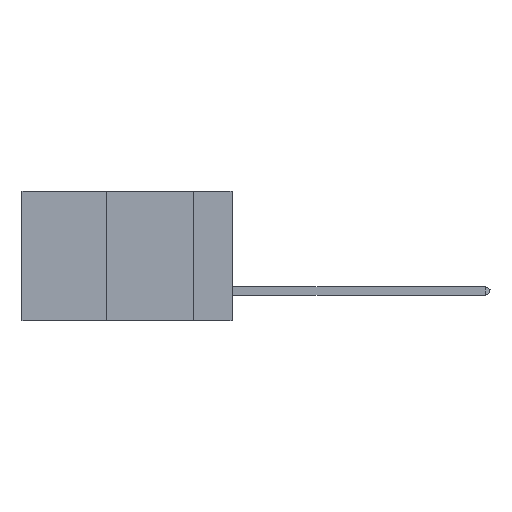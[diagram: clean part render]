
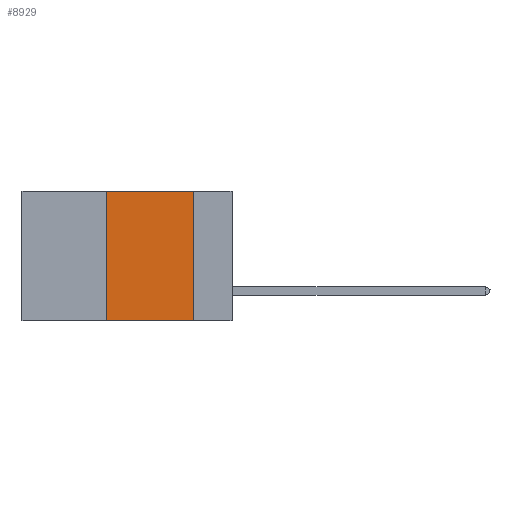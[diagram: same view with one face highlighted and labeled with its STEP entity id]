
A CAD part, left-side view. The second image highlights one B-rep face of the part: STEP entity #8929.
In plain terms, the highlighted planar face has unit normal (-1, 0, 0).
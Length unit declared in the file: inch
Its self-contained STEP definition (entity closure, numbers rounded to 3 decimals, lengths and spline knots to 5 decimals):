
#135 = CARTESIAN_POINT ( 'NONE',  ( 0., 0.36, 0. ) ) ;
#258 = DIRECTION ( 'NONE',  ( 0., 0., 1. ) ) ;
#318 = DIRECTION ( 'NONE',  ( 1., 0., 0. ) ) ;
#398 = VECTOR ( 'NONE', #1254, 39.37008 ) ;
#1254 = DIRECTION ( 'NONE',  ( 0., 0., -1. ) ) ;
#1463 = DIRECTION ( 'NONE',  ( 0., -1., 0. ) ) ;
#1629 = DIRECTION ( 'NONE',  ( 0., -1., 0. ) ) ;
#2200 = VECTOR ( 'NONE', #1629, 39.37008 ) ;
#2343 = ORIENTED_EDGE ( 'NONE', *, *, #4038, .F. ) ;
#2389 = VERTEX_POINT ( 'NONE', #10742 ) ;
#3340 = LINE ( 'NONE', #135, #8206 ) ;
#3611 = CARTESIAN_POINT ( 'NONE',  ( 0., 0.11, 0. ) ) ;
#3669 = VERTEX_POINT ( 'NONE', #8957 ) ;
#4038 = EDGE_CURVE ( 'NONE', #2389, #3669, #3340, .T. ) ;
#4509 = LINE ( 'NONE', #11048, #2200 ) ;
#4709 = AXIS2_PLACEMENT_3D ( 'NONE', #8963, #318, #8006 ) ;
#4723 = ORIENTED_EDGE ( 'NONE', *, *, #5851, .F. ) ;
#4861 = EDGE_LOOP ( 'NONE', ( #4723, #11963, #2343, #10831 ) ) ;
#5778 = EDGE_CURVE ( 'NONE', #3669, #8284, #5887, .T. ) ;
#5851 = EDGE_CURVE ( 'NONE', #8284, #12227, #9805, .T. ) ;
#5887 = LINE ( 'NONE', #7289, #8143 ) ;
#5920 = FACE_OUTER_BOUND ( 'NONE', #4861, .T. ) ;
#6932 = CARTESIAN_POINT ( 'NONE',  ( 0., 0.11, -0.37 ) ) ;
#7289 = CARTESIAN_POINT ( 'NONE',  ( 0., 0.6, 0. ) ) ;
#7802 = CARTESIAN_POINT ( 'NONE',  ( 0., 0.11, 0. ) ) ;
#7961 = PLANE ( 'NONE',  #4709 ) ;
#8006 = DIRECTION ( 'NONE',  ( 0., 0., -1. ) ) ;
#8143 = VECTOR ( 'NONE', #1463, 39.37008 ) ;
#8206 = VECTOR ( 'NONE', #258, 39.37008 ) ;
#8284 = VERTEX_POINT ( 'NONE', #3611 ) ;
#8929 = ADVANCED_FACE ( 'NONE', ( #5920 ), #7961, .F. ) ;
#8957 = CARTESIAN_POINT ( 'NONE',  ( 0., 0.36, 0. ) ) ;
#8963 = CARTESIAN_POINT ( 'NONE',  ( 0., 0.6, 0. ) ) ;
#9805 = LINE ( 'NONE', #7802, #398 ) ;
#10473 = EDGE_CURVE ( 'NONE', #2389, #12227, #4509, .T. ) ;
#10742 = CARTESIAN_POINT ( 'NONE',  ( 0., 0.36, -0.37 ) ) ;
#10831 = ORIENTED_EDGE ( 'NONE', *, *, #10473, .T. ) ;
#11048 = CARTESIAN_POINT ( 'NONE',  ( 0., 0.6, -0.37 ) ) ;
#11963 = ORIENTED_EDGE ( 'NONE', *, *, #5778, .F. ) ;
#12227 = VERTEX_POINT ( 'NONE', #6932 ) ;
